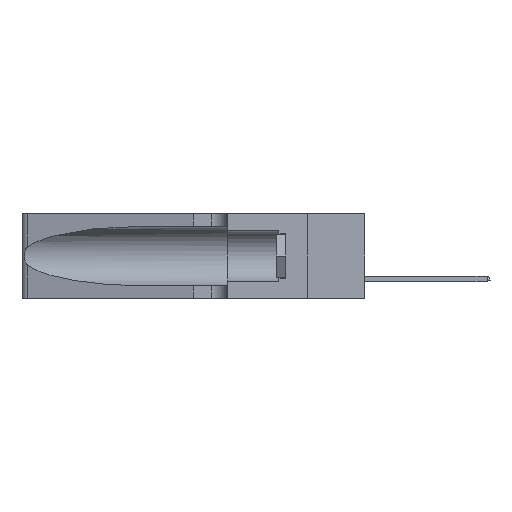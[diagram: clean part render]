
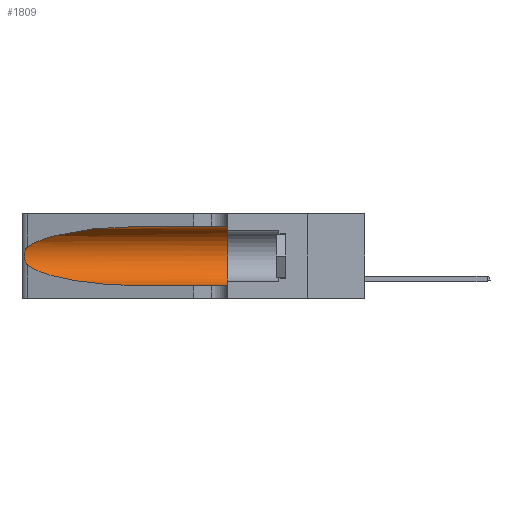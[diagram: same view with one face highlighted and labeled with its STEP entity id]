
A CAD part, left-side view. The second image highlights one B-rep face of the part: STEP entity #1809.
In plain terms, the highlighted cylindrical face has radius 3.308 mm (diameter 6.617 mm), a partial arc.
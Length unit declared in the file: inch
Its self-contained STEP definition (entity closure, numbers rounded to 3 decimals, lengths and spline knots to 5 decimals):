
#792 = EDGE_LOOP ( 'NONE', ( #6033, #2853, #1936, #10203, #3069, #10596 ) ) ;
#1106 = B_SPLINE_CURVE_WITH_KNOTS ( 'NONE', 3,
 ( #11377, #4176, #19655, #15739, #11228, #1280, #14440, #1355, #12841, #3029, #14580, #16241, #6350, #8001 ),
 .UNSPECIFIED., .F., .F.,
 ( 4, 2, 2, 2, 2, 2, 4 ),
 ( 0., 0.00027, 0.00053, 0.00107, 0.0016, 0.00187, 0.00214 ),
 .UNSPECIFIED. ) ;
#1280 = CARTESIAN_POINT ( 'NONE',  ( 0.26018, 1.23835, 0.19895 ) ) ;
#1336 = CARTESIAN_POINT ( 'NONE',  ( 0.1305, 1.61858, 0.185 ) ) ;
#1355 = CARTESIAN_POINT ( 'NONE',  ( 0.26075, 1.23896, 0.178 ) ) ;
#1512 = CARTESIAN_POINT ( 'NONE',  ( 0.1305, 0.35, 0.31525 ) ) ;
#1809 = ADVANCED_FACE ( 'NONE', ( #3572 ), #12610, .F. ) ;
#1936 = ORIENTED_EDGE ( 'NONE', *, *, #6873, .T. ) ;
#2512 = VERTEX_POINT ( 'NONE', #19249 ) ;
#2560 = CARTESIAN_POINT ( 'NONE',  ( 0.18966, 0.96281, 0.31525 ) ) ;
#2668 = VERTEX_POINT ( 'NONE', #7423 ) ;
#2680 = VECTOR ( 'NONE', #8791, 39.37008 ) ;
#2853 = ORIENTED_EDGE ( 'NONE', *, *, #6069, .T. ) ;
#3029 = CARTESIAN_POINT ( 'NONE',  ( 0.25856, 1.23593, 0.16098 ) ) ;
#3069 = ORIENTED_EDGE ( 'NONE', *, *, #17899, .F. ) ;
#3107 = CARTESIAN_POINT ( 'NONE',  ( 0.1305, 0.72297, 0.05475 ) ) ;
#3572 = FACE_OUTER_BOUND ( 'NONE', #792, .T. ) ;
#4176 = CARTESIAN_POINT ( 'NONE',  ( 0.25555, 1.22994, 0.2215 ) ) ;
#4632 = CARTESIAN_POINT ( 'NONE',  ( 0.25487, 1.22718, 0.14631 ) ) ;
#5631 = EDGE_CURVE ( 'NONE', #20917, #6506, #13516, .T. ) ;
#6033 = ORIENTED_EDGE ( 'NONE', *, *, #10545, .T. ) ;
#6069 = EDGE_CURVE ( 'NONE', #19227, #2512, #1106, .T. ) ;
#6166 = CARTESIAN_POINT ( 'NONE',  ( 0.25487, 1.22718, 0.22369 ) ) ;
#6350 = CARTESIAN_POINT ( 'NONE',  ( 0.25555, 1.22993, 0.14849 ) ) ;
#6506 = VERTEX_POINT ( 'NONE', #1512 ) ;
#6639 = DIRECTION ( 'NONE',  ( 0., 1., 0. ) ) ;
#6873 = EDGE_CURVE ( 'NONE', #2512, #8707, #21390, .T. ) ;
#7423 = CARTESIAN_POINT ( 'NONE',  ( 0.1305, 0.35, 0.05475 ) ) ;
#7935 = CARTESIAN_POINT ( 'NONE',  ( 0.1305, 0.72297, 0.05475 ) ) ;
#8001 = CARTESIAN_POINT ( 'NONE',  ( 0.25487, 1.22718, 0.14631 ) ) ;
#8206 = DIRECTION ( 'NONE',  ( 0., -1., 0. ) ) ;
#8707 = VERTEX_POINT ( 'NONE', #3107 ) ;
#8791 = DIRECTION ( 'NONE',  ( 0., -1., 0. ) ) ;
#9508 = CARTESIAN_POINT ( 'NONE',  ( 0.2373, 1.15595, 0.08982 ) ) ;
#10203 = ORIENTED_EDGE ( 'NONE', *, *, #17325, .T. ) ;
#10445 = VECTOR ( 'NONE', #12631, 39.37008 ) ;
#10545 = EDGE_CURVE ( 'NONE', #20917, #19227, #15564, .T. ) ;
#10596 = ORIENTED_EDGE ( 'NONE', *, *, #5631, .F. ) ;
#10913 = CARTESIAN_POINT ( 'NONE',  ( 0.1305, 1.61858, 0.05475 ) ) ;
#11228 = CARTESIAN_POINT ( 'NONE',  ( 0.25854, 1.2359, 0.20912 ) ) ;
#11233 = LINE ( 'NONE', #10913, #10445 ) ;
#11377 = CARTESIAN_POINT ( 'NONE',  ( 0.25487, 1.22718, 0.22369 ) ) ;
#11470 = CARTESIAN_POINT ( 'NONE',  ( 0.1305, 0.72297, 0.31525 ) ) ;
#12423 = CARTESIAN_POINT ( 'NONE',  ( 0.1305, 1.61858, 0.31525 ) ) ;
#12456 = CARTESIAN_POINT ( 'NONE',  ( 0.1305, 0.72297, 0.31525 ) ) ;
#12610 = CYLINDRICAL_SURFACE ( 'NONE', #14372, 0.13025 ) ;
#12631 = DIRECTION ( 'NONE',  ( 0., -1., 0. ) ) ;
#12841 = CARTESIAN_POINT ( 'NONE',  ( 0.26017, 1.23833, 0.17102 ) ) ;
#12894 = DIRECTION ( 'NONE',  ( 0., 0., -1. ) ) ;
#13516 = LINE ( 'NONE', #12423, #2680 ) ;
#14372 = AXIS2_PLACEMENT_3D ( 'NONE', #1336, #8206, #12894 ) ;
#14440 = CARTESIAN_POINT ( 'NONE',  ( 0.26075, 1.23896, 0.19203 ) ) ;
#14580 = CARTESIAN_POINT ( 'NONE',  ( 0.25789, 1.23486, 0.15765 ) ) ;
#15564 =( BOUNDED_CURVE ( )  B_SPLINE_CURVE ( 3, ( #12456, #2560, #15986, #6166 ),
 .UNSPECIFIED., .F., .F. ) 
 B_SPLINE_CURVE_WITH_KNOTS ( ( 4, 4 ),
 ( 1.5708, 2.84003 ),
 .UNSPECIFIED. ) 
 CURVE ( )  GEOMETRIC_REPRESENTATION_ITEM ( )  RATIONAL_B_SPLINE_CURVE ( ( 1., 0.87, 0.87, 1. ) ) 
 REPRESENTATION_ITEM ( '' )  );
#15739 = CARTESIAN_POINT ( 'NONE',  ( 0.25787, 1.23484, 0.2124 ) ) ;
#15928 = AXIS2_PLACEMENT_3D ( 'NONE', #19796, #6639, #20087 ) ;
#15986 = CARTESIAN_POINT ( 'NONE',  ( 0.2373, 1.15595, 0.28018 ) ) ;
#16241 = CARTESIAN_POINT ( 'NONE',  ( 0.25639, 1.23186, 0.15144 ) ) ;
#16958 = CARTESIAN_POINT ( 'NONE',  ( 0.25487, 1.22718, 0.22369 ) ) ;
#17325 = EDGE_CURVE ( 'NONE', #8707, #2668, #11233, .T. ) ;
#17478 = CIRCLE ( 'NONE', #15928, 0.13025 ) ;
#17899 = EDGE_CURVE ( 'NONE', #6506, #2668, #17478, .T. ) ;
#19227 = VERTEX_POINT ( 'NONE', #16958 ) ;
#19249 = CARTESIAN_POINT ( 'NONE',  ( 0.25487, 1.22718, 0.14631 ) ) ;
#19655 = CARTESIAN_POINT ( 'NONE',  ( 0.25639, 1.23184, 0.21858 ) ) ;
#19796 = CARTESIAN_POINT ( 'NONE',  ( 0.1305, 0.35, 0.185 ) ) ;
#20087 = DIRECTION ( 'NONE',  ( 0., 0., 1. ) ) ;
#20917 = VERTEX_POINT ( 'NONE', #11470 ) ;
#21241 = CARTESIAN_POINT ( 'NONE',  ( 0.18966, 0.96281, 0.05475 ) ) ;
#21390 =( BOUNDED_CURVE ( )  B_SPLINE_CURVE ( 3, ( #4632, #9508, #21241, #7935 ),
 .UNSPECIFIED., .F., .T. ) 
 B_SPLINE_CURVE_WITH_KNOTS ( ( 4, 4 ),
 ( 3.44316, 4.71239 ),
 .UNSPECIFIED. ) 
 CURVE ( )  GEOMETRIC_REPRESENTATION_ITEM ( )  RATIONAL_B_SPLINE_CURVE ( ( 1., 0.87, 0.87, 1. ) ) 
 REPRESENTATION_ITEM ( '' )  );
